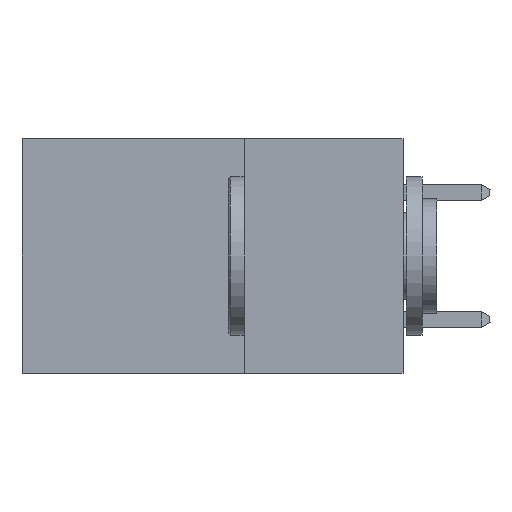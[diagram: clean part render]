
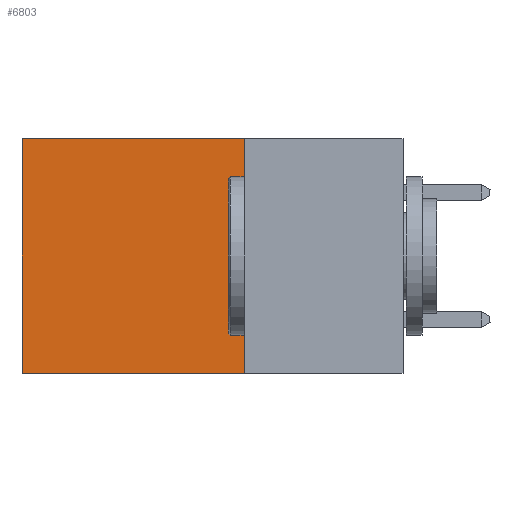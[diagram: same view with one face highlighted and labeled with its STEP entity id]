
A CAD part, left-side view. The second image highlights one B-rep face of the part: STEP entity #6803.
In plain terms, the highlighted planar face has unit normal (-1, 0, 0).
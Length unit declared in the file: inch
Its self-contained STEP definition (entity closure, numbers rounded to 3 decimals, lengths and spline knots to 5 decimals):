
#147 = AXIS2_PLACEMENT_3D ( 'NONE', #897, #6187, #15146 ) ;
#897 = CARTESIAN_POINT ( 'NONE',  ( 0.2875, 0.25, 0. ) ) ;
#1001 = DIRECTION ( 'NONE',  ( 0., 0., -1. ) ) ;
#1196 = LINE ( 'NONE', #1462, #7766 ) ;
#1462 = CARTESIAN_POINT ( 'NONE',  ( 0.2875, 0.25, -0.37 ) ) ;
#1955 = VERTEX_POINT ( 'NONE', #8984 ) ;
#3289 = CARTESIAN_POINT ( 'NONE',  ( 0.2875, 0.25, 0. ) ) ;
#3615 = CARTESIAN_POINT ( 'NONE',  ( 0.2875, 0.25, -0.37 ) ) ;
#3992 = VERTEX_POINT ( 'NONE', #3615 ) ;
#4694 = ORIENTED_EDGE ( 'NONE', *, *, #11765, .T. ) ;
#5030 = EDGE_CURVE ( 'NONE', #9049, #3992, #12502, .T. ) ;
#5930 = ORIENTED_EDGE ( 'NONE', *, *, #11991, .F. ) ;
#6187 = DIRECTION ( 'NONE',  ( 1., 0., 0. ) ) ;
#6218 = ORIENTED_EDGE ( 'NONE', *, *, #10460, .T. ) ;
#6791 = DIRECTION ( 'NONE',  ( 0., 1., 0. ) ) ;
#6803 = ADVANCED_FACE ( 'NONE', ( #16234 ), #13868, .F. ) ;
#7766 = VECTOR ( 'NONE', #6791, 39.37008 ) ;
#8422 = ORIENTED_EDGE ( 'NONE', *, *, #5030, .F. ) ;
#8984 = CARTESIAN_POINT ( 'NONE',  ( 0.2875, 0.6, 0. ) ) ;
#9049 = VERTEX_POINT ( 'NONE', #3289 ) ;
#10460 = EDGE_CURVE ( 'NONE', #9049, #1955, #16380, .T. ) ;
#11205 = CARTESIAN_POINT ( 'NONE',  ( 0.2875, 0.25, 0. ) ) ;
#11352 = VECTOR ( 'NONE', #1001, 39.37008 ) ;
#11765 = EDGE_CURVE ( 'NONE', #1955, #15563, #14763, .T. ) ;
#11991 = EDGE_CURVE ( 'NONE', #3992, #15563, #1196, .T. ) ;
#12221 = EDGE_LOOP ( 'NONE', ( #4694, #5930, #8422, #6218 ) ) ;
#12502 = LINE ( 'NONE', #13648, #15510 ) ;
#12793 = DIRECTION ( 'NONE',  ( 0., 0., -1. ) ) ;
#13648 = CARTESIAN_POINT ( 'NONE',  ( 0.2875, 0.25, 0. ) ) ;
#13868 = PLANE ( 'NONE',  #147 ) ;
#13913 = CARTESIAN_POINT ( 'NONE',  ( 0.2875, 0.6, 0. ) ) ;
#14763 = LINE ( 'NONE', #13913, #11352 ) ;
#15066 = DIRECTION ( 'NONE',  ( 0., 1., 0. ) ) ;
#15146 = DIRECTION ( 'NONE',  ( 0., 0., -1. ) ) ;
#15510 = VECTOR ( 'NONE', #12793, 39.37008 ) ;
#15563 = VERTEX_POINT ( 'NONE', #16658 ) ;
#15592 = VECTOR ( 'NONE', #15066, 39.37008 ) ;
#16234 = FACE_OUTER_BOUND ( 'NONE', #12221, .T. ) ;
#16380 = LINE ( 'NONE', #11205, #15592 ) ;
#16658 = CARTESIAN_POINT ( 'NONE',  ( 0.2875, 0.6, -0.37 ) ) ;
